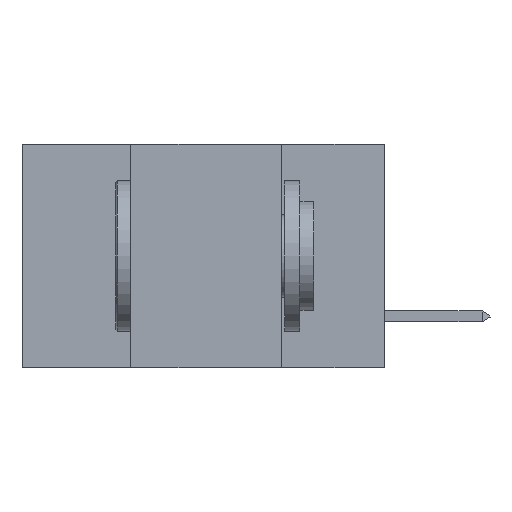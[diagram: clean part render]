
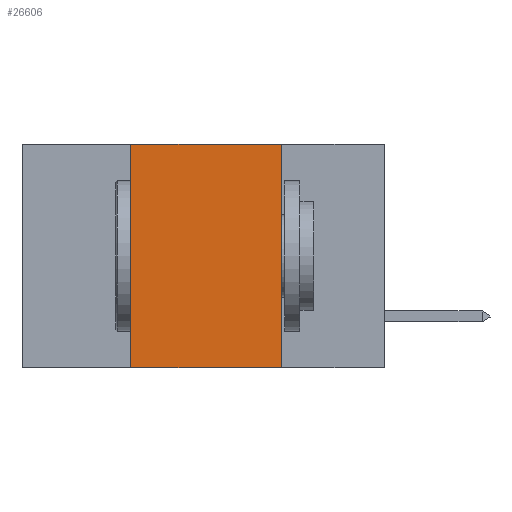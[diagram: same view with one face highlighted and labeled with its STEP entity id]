
A CAD part, left-side view. The second image highlights one B-rep face of the part: STEP entity #26606.
In plain terms, the highlighted planar face has unit normal (-1, 0, 0).
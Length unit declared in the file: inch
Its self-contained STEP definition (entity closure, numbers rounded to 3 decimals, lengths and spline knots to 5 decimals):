
#109 = ORIENTED_EDGE ( 'NONE', *, *, #22016, .F. ) ;
#1702 = DIRECTION ( 'NONE',  ( 0., 0., 1. ) ) ;
#2142 = FACE_OUTER_BOUND ( 'NONE', #11783, .T. ) ;
#2790 = VERTEX_POINT ( 'NONE', #21575 ) ;
#4049 = CARTESIAN_POINT ( 'NONE',  ( 0., 0.42, 0. ) ) ;
#4157 = CARTESIAN_POINT ( 'NONE',  ( 0., 0.17, 0. ) ) ;
#6381 = CARTESIAN_POINT ( 'NONE',  ( 0., 0.6, 0. ) ) ;
#6898 = EDGE_CURVE ( 'NONE', #8483, #2790, #7090, .T. ) ;
#7090 = LINE ( 'NONE', #34361, #34066 ) ;
#7309 = EDGE_CURVE ( 'NONE', #8483, #20201, #25997, .T. ) ;
#7764 = VERTEX_POINT ( 'NONE', #4157 ) ;
#8483 = VERTEX_POINT ( 'NONE', #27431 ) ;
#9155 = VECTOR ( 'NONE', #1702, 39.37008 ) ;
#10034 = LINE ( 'NONE', #6381, #34884 ) ;
#10290 = DIRECTION ( 'NONE',  ( 1., 0., 0. ) ) ;
#11783 = EDGE_LOOP ( 'NONE', ( #31589, #109, #11844, #13965 ) ) ;
#11844 = ORIENTED_EDGE ( 'NONE', *, *, #7309, .F. ) ;
#12047 = AXIS2_PLACEMENT_3D ( 'NONE', #18834, #10290, #26720 ) ;
#13932 = CARTESIAN_POINT ( 'NONE',  ( 0., 0.42, 0. ) ) ;
#13965 = ORIENTED_EDGE ( 'NONE', *, *, #6898, .T. ) ;
#16037 = PLANE ( 'NONE',  #12047 ) ;
#18834 = CARTESIAN_POINT ( 'NONE',  ( 0., 0.6, 0. ) ) ;
#19707 = CARTESIAN_POINT ( 'NONE',  ( 0., 0.17, 0. ) ) ;
#20201 = VERTEX_POINT ( 'NONE', #13932 ) ;
#21575 = CARTESIAN_POINT ( 'NONE',  ( 0., 0.17, -0.37 ) ) ;
#22016 = EDGE_CURVE ( 'NONE', #20201, #7764, #10034, .T. ) ;
#24582 = EDGE_CURVE ( 'NONE', #7764, #2790, #32655, .T. ) ;
#25997 = LINE ( 'NONE', #4049, #9155 ) ;
#26606 = ADVANCED_FACE ( 'NONE', ( #2142 ), #16037, .F. ) ;
#26720 = DIRECTION ( 'NONE',  ( 0., 0., -1. ) ) ;
#27162 = VECTOR ( 'NONE', #30191, 39.37008 ) ;
#27431 = CARTESIAN_POINT ( 'NONE',  ( 0., 0.42, -0.37 ) ) ;
#28064 = DIRECTION ( 'NONE',  ( 0., -1., 0. ) ) ;
#28669 = DIRECTION ( 'NONE',  ( 0., -1., 0. ) ) ;
#30191 = DIRECTION ( 'NONE',  ( 0., 0., -1. ) ) ;
#31589 = ORIENTED_EDGE ( 'NONE', *, *, #24582, .F. ) ;
#32655 = LINE ( 'NONE', #19707, #27162 ) ;
#34066 = VECTOR ( 'NONE', #28669, 39.37008 ) ;
#34361 = CARTESIAN_POINT ( 'NONE',  ( 0., 0.6, -0.37 ) ) ;
#34884 = VECTOR ( 'NONE', #28064, 39.37008 ) ;
